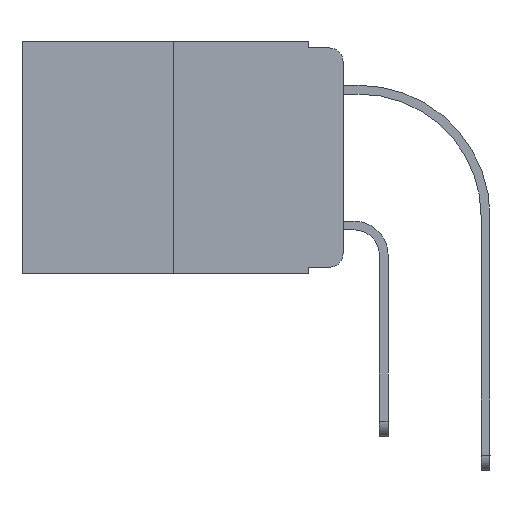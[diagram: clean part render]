
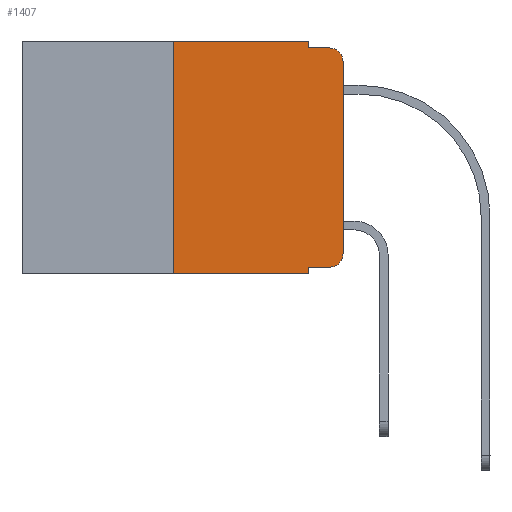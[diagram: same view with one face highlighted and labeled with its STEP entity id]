
A CAD part, left-side view. The second image highlights one B-rep face of the part: STEP entity #1407.
In plain terms, the highlighted planar face has unit normal (-1, 0, 0).
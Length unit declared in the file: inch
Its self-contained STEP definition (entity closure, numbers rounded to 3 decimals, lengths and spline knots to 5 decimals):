
#88 = CARTESIAN_POINT ( 'NONE',  ( 0., 0.473, 0. ) ) ;
#237 = DIRECTION ( 'NONE',  ( 1., 0., 0. ) ) ;
#519 = VECTOR ( 'NONE', #5517, 39.37008 ) ;
#620 = CARTESIAN_POINT ( 'NONE',  ( 0., 0.02, -0.01 ) ) ;
#962 = CARTESIAN_POINT ( 'NONE',  ( 0., 0.051, -0.01 ) ) ;
#1122 = CARTESIAN_POINT ( 'NONE',  ( 0., 0.02, -0.333 ) ) ;
#1137 = LINE ( 'NONE', #12452, #11864 ) ;
#1181 = LINE ( 'NONE', #4478, #5339 ) ;
#1341 = DIRECTION ( 'NONE',  ( 0., 0., -1. ) ) ;
#1407 = ADVANCED_FACE ( 'NONE', ( #14051 ), #13067, .F. ) ;
#1431 = ORIENTED_EDGE ( 'NONE', *, *, #4944, .T. ) ;
#1945 = ORIENTED_EDGE ( 'NONE', *, *, #14652, .F. ) ;
#2015 = VERTEX_POINT ( 'NONE', #14323 ) ;
#2050 = AXIS2_PLACEMENT_3D ( 'NONE', #88, #237, #12919 ) ;
#2228 = EDGE_CURVE ( 'NONE', #2250, #2015, #13023, .T. ) ;
#2250 = VERTEX_POINT ( 'NONE', #1122 ) ;
#2782 = CARTESIAN_POINT ( 'NONE',  ( 0., 0.051, -0.01 ) ) ;
#3061 = LINE ( 'NONE', #9785, #9287 ) ;
#3560 = LINE ( 'NONE', #11738, #7008 ) ;
#3731 = EDGE_CURVE ( 'NONE', #10591, #3934, #1137, .T. ) ;
#3774 = AXIS2_PLACEMENT_3D ( 'NONE', #13393, #14523, #5073 ) ;
#3934 = VERTEX_POINT ( 'NONE', #6395 ) ;
#3940 = VERTEX_POINT ( 'NONE', #9315 ) ;
#4002 = LINE ( 'NONE', #8881, #12710 ) ;
#4345 = EDGE_CURVE ( 'NONE', #3934, #9778, #3560, .T. ) ;
#4370 = CARTESIAN_POINT ( 'NONE',  ( 0., 0.051, 0. ) ) ;
#4478 = CARTESIAN_POINT ( 'NONE',  ( 0., 0.051, -0.333 ) ) ;
#4944 = EDGE_CURVE ( 'NONE', #2015, #10624, #7659, .T. ) ;
#5073 = DIRECTION ( 'NONE',  ( 0., 0., -1. ) ) ;
#5339 = VECTOR ( 'NONE', #5847, 39.37008 ) ;
#5517 = DIRECTION ( 'NONE',  ( 0., 0., 1. ) ) ;
#5595 = VECTOR ( 'NONE', #10660, 39.37008 ) ;
#5799 = DIRECTION ( 'NONE',  ( 0., 0., 1. ) ) ;
#5847 = DIRECTION ( 'NONE',  ( 0., -1., 0. ) ) ;
#6256 = ORIENTED_EDGE ( 'NONE', *, *, #4345, .F. ) ;
#6375 = EDGE_CURVE ( 'NONE', #9778, #11092, #14735, .T. ) ;
#6395 = CARTESIAN_POINT ( 'NONE',  ( 0., 0.25, 0. ) ) ;
#6495 = CARTESIAN_POINT ( 'NONE',  ( 0., 0., -0.03 ) ) ;
#6914 = CARTESIAN_POINT ( 'NONE',  ( 0., 0.051, 0. ) ) ;
#7008 = VECTOR ( 'NONE', #8452, 39.37008 ) ;
#7064 = EDGE_LOOP ( 'NONE', ( #1431, #9619, #11589, #12703, #6256, #10712, #7389, #1945, #10018, #11428 ) ) ;
#7326 = CARTESIAN_POINT ( 'NONE',  ( 0., 0.051, -0.343 ) ) ;
#7350 = EDGE_CURVE ( 'NONE', #10624, #11996, #8425, .T. ) ;
#7389 = ORIENTED_EDGE ( 'NONE', *, *, #12065, .T. ) ;
#7659 = LINE ( 'NONE', #13601, #519 ) ;
#8425 = CIRCLE ( 'NONE', #3774, 0.02 ) ;
#8452 = DIRECTION ( 'NONE',  ( 0., -1., 0. ) ) ;
#8512 = DIRECTION ( 'NONE',  ( 0., 0., -1. ) ) ;
#8784 = CARTESIAN_POINT ( 'NONE',  ( 0., 0.25, -0.343 ) ) ;
#8881 = CARTESIAN_POINT ( 'NONE',  ( 0., 0.051, 0. ) ) ;
#9287 = VECTOR ( 'NONE', #11014, 39.37008 ) ;
#9315 = CARTESIAN_POINT ( 'NONE',  ( 0., 0.051, -0.333 ) ) ;
#9373 = DIRECTION ( 'NONE',  ( -1., 0., 0. ) ) ;
#9619 = ORIENTED_EDGE ( 'NONE', *, *, #7350, .T. ) ;
#9778 = VERTEX_POINT ( 'NONE', #6914 ) ;
#9785 = CARTESIAN_POINT ( 'NONE',  ( 0., 0.473, -0.343 ) ) ;
#9896 = EDGE_CURVE ( 'NONE', #3940, #2250, #1181, .T. ) ;
#10018 = ORIENTED_EDGE ( 'NONE', *, *, #9896, .T. ) ;
#10108 = DIRECTION ( 'NONE',  ( 0., 0., -1. ) ) ;
#10591 = VERTEX_POINT ( 'NONE', #8784 ) ;
#10624 = VERTEX_POINT ( 'NONE', #6495 ) ;
#10660 = DIRECTION ( 'NONE',  ( 0., -1., 0. ) ) ;
#10712 = ORIENTED_EDGE ( 'NONE', *, *, #3731, .F. ) ;
#11014 = DIRECTION ( 'NONE',  ( 0., -1., 0. ) ) ;
#11092 = VERTEX_POINT ( 'NONE', #962 ) ;
#11250 = EDGE_CURVE ( 'NONE', #11092, #11996, #14150, .T. ) ;
#11428 = ORIENTED_EDGE ( 'NONE', *, *, #2228, .T. ) ;
#11589 = ORIENTED_EDGE ( 'NONE', *, *, #11250, .F. ) ;
#11738 = CARTESIAN_POINT ( 'NONE',  ( 0., 0.473, 0. ) ) ;
#11820 = CARTESIAN_POINT ( 'NONE',  ( 0., 0.02, -0.313 ) ) ;
#11864 = VECTOR ( 'NONE', #5799, 39.37008 ) ;
#11996 = VERTEX_POINT ( 'NONE', #620 ) ;
#12065 = EDGE_CURVE ( 'NONE', #10591, #14928, #3061, .T. ) ;
#12452 = CARTESIAN_POINT ( 'NONE',  ( 0., 0.25, 0. ) ) ;
#12703 = ORIENTED_EDGE ( 'NONE', *, *, #6375, .F. ) ;
#12710 = VECTOR ( 'NONE', #8512, 39.37008 ) ;
#12919 = DIRECTION ( 'NONE',  ( 0., 0., -1. ) ) ;
#13023 = CIRCLE ( 'NONE', #14951, 0.02 ) ;
#13067 = PLANE ( 'NONE',  #2050 ) ;
#13393 = CARTESIAN_POINT ( 'NONE',  ( 0., 0.02, -0.03 ) ) ;
#13499 = VECTOR ( 'NONE', #10108, 39.37008 ) ;
#13601 = CARTESIAN_POINT ( 'NONE',  ( 0., 0., 0. ) ) ;
#14051 = FACE_OUTER_BOUND ( 'NONE', #7064, .T. ) ;
#14150 = LINE ( 'NONE', #2782, #5595 ) ;
#14323 = CARTESIAN_POINT ( 'NONE',  ( 0., 0., -0.313 ) ) ;
#14523 = DIRECTION ( 'NONE',  ( -1., 0., 0. ) ) ;
#14652 = EDGE_CURVE ( 'NONE', #3940, #14928, #4002, .T. ) ;
#14735 = LINE ( 'NONE', #4370, #13499 ) ;
#14928 = VERTEX_POINT ( 'NONE', #7326 ) ;
#14951 = AXIS2_PLACEMENT_3D ( 'NONE', #11820, #9373, #1341 ) ;
